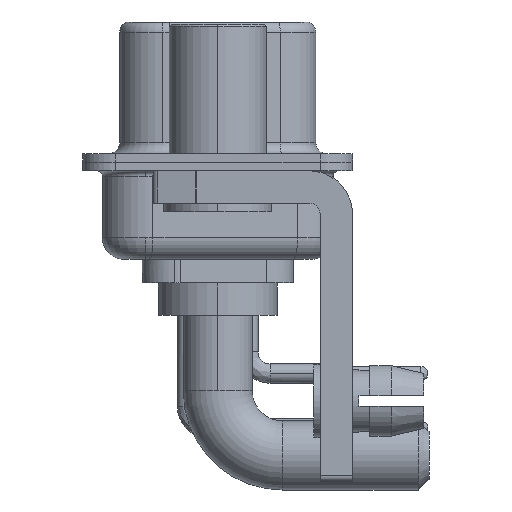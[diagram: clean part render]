
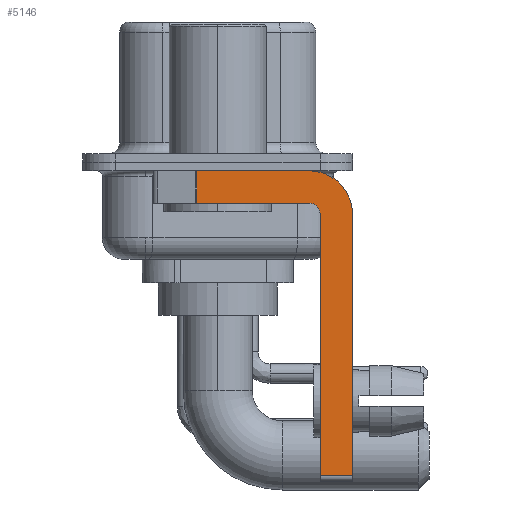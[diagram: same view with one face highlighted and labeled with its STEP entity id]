
A CAD part, left-side view. The second image highlights one B-rep face of the part: STEP entity #5146.
In plain terms, the highlighted planar face has unit normal (-1, 0, 0).
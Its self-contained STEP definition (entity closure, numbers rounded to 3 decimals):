
#80 = CARTESIAN_POINT ( 'NONE',  ( -2.9, -4.75, -2.4 ) ) ;
#311 = VECTOR ( 'NONE', #11593, 1000. ) ;
#497 = DIRECTION ( 'NONE',  ( 0., -1., 0. ) ) ;
#1107 = CIRCLE ( 'NONE', #21760, 2. ) ;
#1224 = EDGE_CURVE ( 'NONE', #24499, #10153, #15536, .T. ) ;
#2285 = ORIENTED_EDGE ( 'NONE', *, *, #10995, .T. ) ;
#2342 = AXIS2_PLACEMENT_3D ( 'NONE', #13874, #25034, #13748 ) ;
#3422 = DIRECTION ( 'NONE',  ( 0., 0., -1. ) ) ;
#3868 = CARTESIAN_POINT ( 'NONE',  ( -2.9, 0.978, -1.9 ) ) ;
#4078 = ORIENTED_EDGE ( 'NONE', *, *, #17375, .F. ) ;
#4111 = CARTESIAN_POINT ( 'NONE',  ( -2.9, 0.978, -1.9 ) ) ;
#5146 = ADVANCED_FACE ( 'NONE', ( #16383 ), #10923, .F. ) ;
#6262 = CARTESIAN_POINT ( 'NONE',  ( -2.9, -6.25, -14.55 ) ) ;
#7322 = EDGE_CURVE ( 'NONE', #24499, #12871, #24967, .T. ) ;
#9023 = ORIENTED_EDGE ( 'NONE', *, *, #1224, .T. ) ;
#9191 = CARTESIAN_POINT ( 'NONE',  ( -2.9, -4.25, -14.55 ) ) ;
#9218 = CIRCLE ( 'NONE', #2342, 0.5 ) ;
#10011 = LINE ( 'NONE', #10725, #20789 ) ;
#10153 = VERTEX_POINT ( 'NONE', #6262 ) ;
#10725 = CARTESIAN_POINT ( 'NONE',  ( -2.9, 3., -0.4 ) ) ;
#10843 = VECTOR ( 'NONE', #25039, 1000. ) ;
#10919 = EDGE_CURVE ( 'NONE', #12871, #21054, #9218, .T. ) ;
#10923 = PLANE ( 'NONE',  #24950 ) ;
#10995 = EDGE_CURVE ( 'NONE', #20432, #13251, #15531, .T. ) ;
#11021 = VERTEX_POINT ( 'NONE', #12591 ) ;
#11048 = DIRECTION ( 'NONE',  ( 0., 0., -1. ) ) ;
#11264 = ORIENTED_EDGE ( 'NONE', *, *, #7322, .F. ) ;
#11393 = VERTEX_POINT ( 'NONE', #14565 ) ;
#11593 = DIRECTION ( 'NONE',  ( 0., 0., -1. ) ) ;
#11655 = CARTESIAN_POINT ( 'NONE',  ( -2.9, -4.75, -14.8 ) ) ;
#11845 = ORIENTED_EDGE ( 'NONE', *, *, #20296, .F. ) ;
#12591 = CARTESIAN_POINT ( 'NONE',  ( -2.9, -4.25, -0.4 ) ) ;
#12871 = VERTEX_POINT ( 'NONE', #80 ) ;
#12949 = DIRECTION ( 'NONE',  ( 1., 0., 0. ) ) ;
#13249 = CARTESIAN_POINT ( 'NONE',  ( -2.9, 0.978, -0.4 ) ) ;
#13251 = VERTEX_POINT ( 'NONE', #4111 ) ;
#13748 = DIRECTION ( 'NONE',  ( 0., 0., 1. ) ) ;
#13874 = CARTESIAN_POINT ( 'NONE',  ( -2.9, -4.25, -2.4 ) ) ;
#14565 = CARTESIAN_POINT ( 'NONE',  ( -2.9, -6.25, -2.4 ) ) ;
#15352 = DIRECTION ( 'NONE',  ( 0., 0., 1. ) ) ;
#15531 = LINE ( 'NONE', #3868, #311 ) ;
#15536 = LINE ( 'NONE', #9191, #10843 ) ;
#15699 = ORIENTED_EDGE ( 'NONE', *, *, #23737, .F. ) ;
#16383 = FACE_OUTER_BOUND ( 'NONE', #22271, .T. ) ;
#16597 = EDGE_CURVE ( 'NONE', #21054, #13251, #23749, .T. ) ;
#17289 = CARTESIAN_POINT ( 'NONE',  ( -2.9, -4.25, -2.4 ) ) ;
#17347 = VECTOR ( 'NONE', #15352, 1000. ) ;
#17375 = EDGE_CURVE ( 'NONE', #11393, #10153, #17841, .T. ) ;
#17841 = LINE ( 'NONE', #19026, #23577 ) ;
#18187 = DIRECTION ( 'NONE',  ( 0., 1., 0. ) ) ;
#18480 = CARTESIAN_POINT ( 'NONE',  ( -2.9, -4.25, -1.9 ) ) ;
#19026 = CARTESIAN_POINT ( 'NONE',  ( -2.9, -6.25, -2.4 ) ) ;
#19063 = DIRECTION ( 'NONE',  ( 1., 0., 0. ) ) ;
#19668 = ORIENTED_EDGE ( 'NONE', *, *, #10919, .F. ) ;
#19930 = VECTOR ( 'NONE', #18187, 1000. ) ;
#20084 = CARTESIAN_POINT ( 'NONE',  ( -2.9, -4.25, -1.9 ) ) ;
#20296 = EDGE_CURVE ( 'NONE', #20432, #11021, #10011, .T. ) ;
#20432 = VERTEX_POINT ( 'NONE', #13249 ) ;
#20789 = VECTOR ( 'NONE', #497, 1000. ) ;
#21054 = VERTEX_POINT ( 'NONE', #18480 ) ;
#21760 = AXIS2_PLACEMENT_3D ( 'NONE', #17289, #19063, #23354 ) ;
#22271 = EDGE_LOOP ( 'NONE', ( #11845, #2285, #22912, #19668, #11264, #9023, #4078, #15699 ) ) ;
#22334 = CARTESIAN_POINT ( 'NONE',  ( -2.9, -4.25, -2.4 ) ) ;
#22418 = CARTESIAN_POINT ( 'NONE',  ( -2.9, -4.75, -14.55 ) ) ;
#22912 = ORIENTED_EDGE ( 'NONE', *, *, #16597, .F. ) ;
#23354 = DIRECTION ( 'NONE',  ( 0., 0., -1. ) ) ;
#23577 = VECTOR ( 'NONE', #3422, 1000. ) ;
#23737 = EDGE_CURVE ( 'NONE', #11021, #11393, #1107, .T. ) ;
#23749 = LINE ( 'NONE', #20084, #19930 ) ;
#24499 = VERTEX_POINT ( 'NONE', #22418 ) ;
#24950 = AXIS2_PLACEMENT_3D ( 'NONE', #22334, #12949, #11048 ) ;
#24967 = LINE ( 'NONE', #11655, #17347 ) ;
#25034 = DIRECTION ( 'NONE',  ( -1., 0., 0. ) ) ;
#25039 = DIRECTION ( 'NONE',  ( 0., -1., 0. ) ) ;
